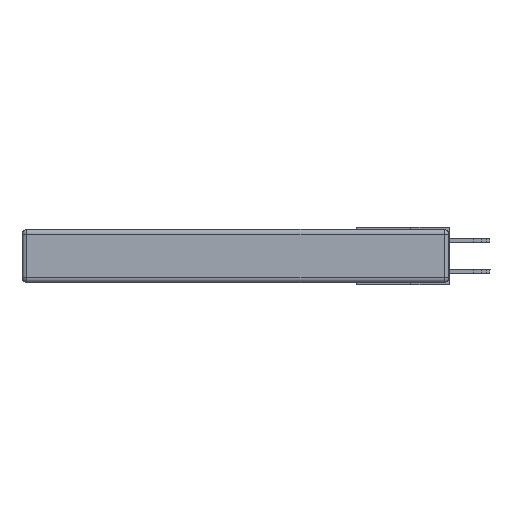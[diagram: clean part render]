
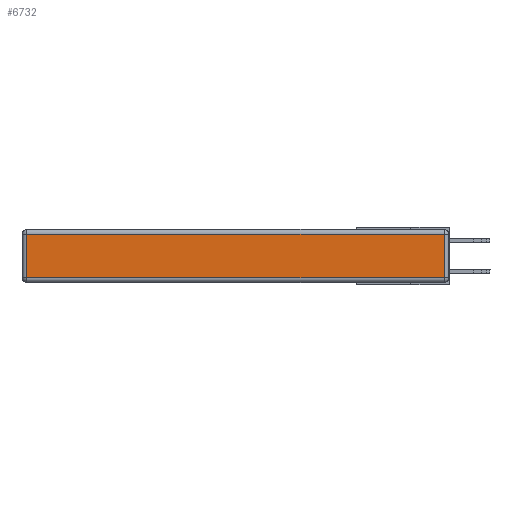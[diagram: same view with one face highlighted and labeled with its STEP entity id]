
A CAD part, left-side view. The second image highlights one B-rep face of the part: STEP entity #6732.
In plain terms, the highlighted planar face has unit normal (-1, 0, 0).
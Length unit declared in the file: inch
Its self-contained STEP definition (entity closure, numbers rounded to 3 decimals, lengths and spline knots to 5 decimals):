
#1035 = CARTESIAN_POINT ( 'NONE',  ( 0., 2.72, -0.343 ) ) ;
#2056 = CARTESIAN_POINT ( 'NONE',  ( 0., 0.03, -0.03 ) ) ;
#2145 = ORIENTED_EDGE ( 'NONE', *, *, #13096, .T. ) ;
#3168 = DIRECTION ( 'NONE',  ( 0., 0., -1. ) ) ;
#3342 = VECTOR ( 'NONE', #3168, 39.37008 ) ;
#3748 = DIRECTION ( 'NONE',  ( 0., -1., 0. ) ) ;
#3832 = VECTOR ( 'NONE', #16973, 39.37008 ) ;
#3847 = AXIS2_PLACEMENT_3D ( 'NONE', #9553, #26392, #22471 ) ;
#4765 = CARTESIAN_POINT ( 'NONE',  ( 0., 0.03, -0.343 ) ) ;
#4829 = EDGE_CURVE ( 'NONE', #27143, #24582, #22375, .T. ) ;
#5502 = ORIENTED_EDGE ( 'NONE', *, *, #19640, .T. ) ;
#6009 = LINE ( 'NONE', #1035, #3342 ) ;
#6732 = ADVANCED_FACE ( 'NONE', ( #17924 ), #7627, .T. ) ;
#7627 = PLANE ( 'NONE',  #3847 ) ;
#8222 = ORIENTED_EDGE ( 'NONE', *, *, #10516, .T. ) ;
#9165 = DIRECTION ( 'NONE',  ( 0., 0., 1. ) ) ;
#9518 = CARTESIAN_POINT ( 'NONE',  ( 0., 2.72, -0.03 ) ) ;
#9553 = CARTESIAN_POINT ( 'NONE',  ( 0., 0., -0.343 ) ) ;
#10516 = EDGE_CURVE ( 'NONE', #19422, #17308, #18175, .T. ) ;
#11184 = LINE ( 'NONE', #4765, #16854 ) ;
#12528 = VECTOR ( 'NONE', #3748, 39.37008 ) ;
#13096 = EDGE_CURVE ( 'NONE', #17308, #27143, #11184, .T. ) ;
#16854 = VECTOR ( 'NONE', #9165, 39.37008 ) ;
#16973 = DIRECTION ( 'NONE',  ( 0., 1., 0. ) ) ;
#17308 = VERTEX_POINT ( 'NONE', #26720 ) ;
#17924 = FACE_OUTER_BOUND ( 'NONE', #25368, .T. ) ;
#18175 = LINE ( 'NONE', #25228, #12528 ) ;
#18916 = CARTESIAN_POINT ( 'NONE',  ( 0., 2.72, -0.313 ) ) ;
#19422 = VERTEX_POINT ( 'NONE', #18916 ) ;
#19640 = EDGE_CURVE ( 'NONE', #24582, #19422, #6009, .T. ) ;
#21042 = ORIENTED_EDGE ( 'NONE', *, *, #4829, .T. ) ;
#22375 = LINE ( 'NONE', #27329, #3832 ) ;
#22471 = DIRECTION ( 'NONE',  ( 0., 0., 1. ) ) ;
#24582 = VERTEX_POINT ( 'NONE', #9518 ) ;
#25228 = CARTESIAN_POINT ( 'NONE',  ( 0., 0., -0.313 ) ) ;
#25368 = EDGE_LOOP ( 'NONE', ( #8222, #2145, #21042, #5502 ) ) ;
#26392 = DIRECTION ( 'NONE',  ( -1., 0., 0. ) ) ;
#26720 = CARTESIAN_POINT ( 'NONE',  ( 0., 0.03, -0.313 ) ) ;
#27143 = VERTEX_POINT ( 'NONE', #2056 ) ;
#27329 = CARTESIAN_POINT ( 'NONE',  ( 0., 2.75, -0.03 ) ) ;
